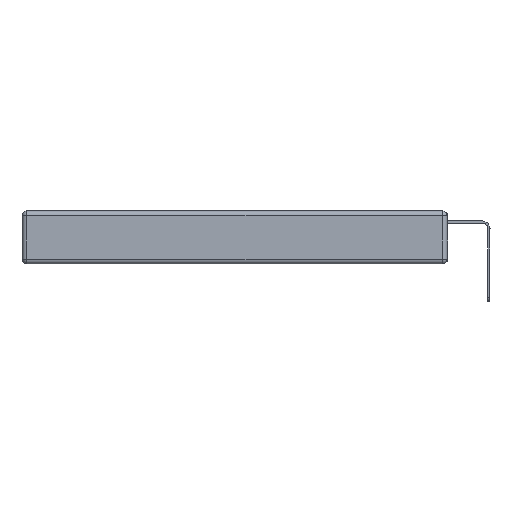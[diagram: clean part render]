
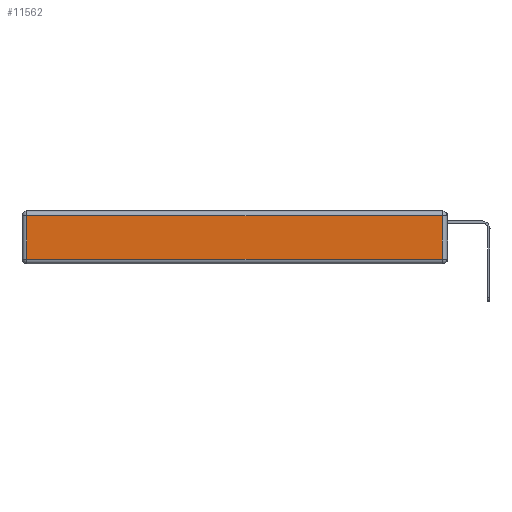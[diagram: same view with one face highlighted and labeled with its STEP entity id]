
A CAD part, left-side view. The second image highlights one B-rep face of the part: STEP entity #11562.
In plain terms, the highlighted planar face has unit normal (-1, 0, 0).
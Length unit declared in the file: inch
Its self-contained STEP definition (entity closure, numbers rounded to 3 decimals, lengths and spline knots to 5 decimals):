
#634 = VERTEX_POINT ( 'NONE', #2549 ) ;
#661 = DIRECTION ( 'NONE',  ( 0., 1., 0. ) ) ;
#827 = EDGE_CURVE ( 'NONE', #15871, #1962, #15970, .T. ) ;
#1510 = VERTEX_POINT ( 'NONE', #9712 ) ;
#1674 = DIRECTION ( 'NONE',  ( 0., -1., 0. ) ) ;
#1962 = VERTEX_POINT ( 'NONE', #9945 ) ;
#2549 = CARTESIAN_POINT ( 'NONE',  ( 0., 0.03, -0.03 ) ) ;
#3412 = LINE ( 'NONE', #14896, #5162 ) ;
#3451 = CARTESIAN_POINT ( 'NONE',  ( 0., 0., -0.343 ) ) ;
#3903 = EDGE_CURVE ( 'NONE', #1962, #634, #3412, .T. ) ;
#5162 = VECTOR ( 'NONE', #6170, 39.37008 ) ;
#5911 = PLANE ( 'NONE',  #11243 ) ;
#6170 = DIRECTION ( 'NONE',  ( 0., 0., 1. ) ) ;
#7196 = CARTESIAN_POINT ( 'NONE',  ( 0., 2.72, -0.343 ) ) ;
#8145 = ORIENTED_EDGE ( 'NONE', *, *, #8486, .T. ) ;
#8410 = DIRECTION ( 'NONE',  ( 0., 0., 1. ) ) ;
#8486 = EDGE_CURVE ( 'NONE', #634, #1510, #11817, .T. ) ;
#9146 = CARTESIAN_POINT ( 'NONE',  ( 0., 0., -0.313 ) ) ;
#9712 = CARTESIAN_POINT ( 'NONE',  ( 0., 2.72, -0.03 ) ) ;
#9868 = EDGE_CURVE ( 'NONE', #1510, #15871, #14410, .T. ) ;
#9945 = CARTESIAN_POINT ( 'NONE',  ( 0., 0.03, -0.313 ) ) ;
#10611 = FACE_OUTER_BOUND ( 'NONE', #12971, .T. ) ;
#10808 = ORIENTED_EDGE ( 'NONE', *, *, #827, .T. ) ;
#11243 = AXIS2_PLACEMENT_3D ( 'NONE', #3451, #13281, #8410 ) ;
#11336 = CARTESIAN_POINT ( 'NONE',  ( 0., 2.72, -0.313 ) ) ;
#11562 = ADVANCED_FACE ( 'NONE', ( #10611 ), #5911, .T. ) ;
#11817 = LINE ( 'NONE', #12952, #12016 ) ;
#12016 = VECTOR ( 'NONE', #661, 39.37008 ) ;
#12270 = DIRECTION ( 'NONE',  ( 0., 0., -1. ) ) ;
#12952 = CARTESIAN_POINT ( 'NONE',  ( 0., 2.75, -0.03 ) ) ;
#12971 = EDGE_LOOP ( 'NONE', ( #10808, #14487, #8145, #15491 ) ) ;
#13281 = DIRECTION ( 'NONE',  ( -1., 0., 0. ) ) ;
#13478 = VECTOR ( 'NONE', #1674, 39.37008 ) ;
#14204 = VECTOR ( 'NONE', #12270, 39.37008 ) ;
#14410 = LINE ( 'NONE', #7196, #14204 ) ;
#14487 = ORIENTED_EDGE ( 'NONE', *, *, #3903, .T. ) ;
#14896 = CARTESIAN_POINT ( 'NONE',  ( 0., 0.03, -0.343 ) ) ;
#15491 = ORIENTED_EDGE ( 'NONE', *, *, #9868, .T. ) ;
#15871 = VERTEX_POINT ( 'NONE', #11336 ) ;
#15970 = LINE ( 'NONE', #9146, #13478 ) ;
